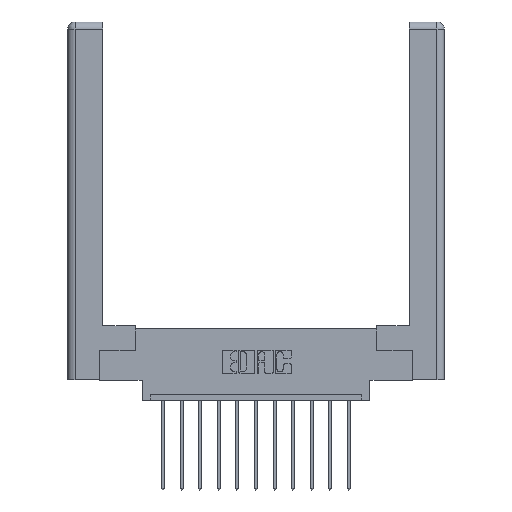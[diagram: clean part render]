
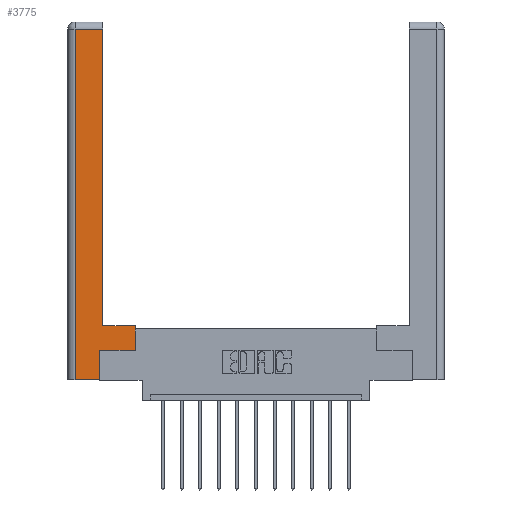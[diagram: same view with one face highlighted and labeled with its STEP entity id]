
A CAD part, top view. The second image highlights one B-rep face of the part: STEP entity #3775.
In plain terms, the highlighted planar face has unit normal (0, 0, 1).
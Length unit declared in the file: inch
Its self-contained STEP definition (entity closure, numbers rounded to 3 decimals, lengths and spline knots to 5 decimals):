
#178 = CARTESIAN_POINT ( 'NONE',  ( 0.295, 2.94, 0. ) ) ;
#1182 = EDGE_CURVE ( 'NONE', #5947, #13692, #11246, .T. ) ;
#1203 = CARTESIAN_POINT ( 'NONE',  ( 0.565, 0.45, 0. ) ) ;
#1439 = CARTESIAN_POINT ( 'NONE',  ( 0.265, 0., 0. ) ) ;
#1519 = FACE_OUTER_BOUND ( 'NONE', #7965, .T. ) ;
#1564 = LINE ( 'NONE', #8539, #3560 ) ;
#1913 = EDGE_CURVE ( 'NONE', #3575, #5947, #8851, .T. ) ;
#1918 = CARTESIAN_POINT ( 'NONE',  ( 0.265, 0.245, 0. ) ) ;
#1952 = VECTOR ( 'NONE', #10999, 39.37008 ) ;
#2088 = VECTOR ( 'NONE', #14551, 39.37008 ) ;
#2549 = VERTEX_POINT ( 'NONE', #10469 ) ;
#3560 = VECTOR ( 'NONE', #7315, 39.37008 ) ;
#3575 = VERTEX_POINT ( 'NONE', #5345 ) ;
#3697 = ORIENTED_EDGE ( 'NONE', *, *, #1182, .T. ) ;
#3775 = ADVANCED_FACE ( 'NONE', ( #1519 ), #8962, .F. ) ;
#3883 = CARTESIAN_POINT ( 'NONE',  ( 0.0615, 0., 0. ) ) ;
#4097 = ORIENTED_EDGE ( 'NONE', *, *, #12690, .T. ) ;
#4231 = VECTOR ( 'NONE', #7386, 39.37008 ) ;
#4236 = DIRECTION ( 'NONE',  ( 0., 1., 0. ) ) ;
#4328 = CARTESIAN_POINT ( 'NONE',  ( 0., 0., 0. ) ) ;
#4984 = LINE ( 'NONE', #7531, #2088 ) ;
#5345 = CARTESIAN_POINT ( 'NONE',  ( 0.265, 0.245, 0. ) ) ;
#5398 = CARTESIAN_POINT ( 'NONE',  ( 0.565, 0.45, 0. ) ) ;
#5839 = EDGE_CURVE ( 'NONE', #7950, #2549, #13059, .T. ) ;
#5947 = VERTEX_POINT ( 'NONE', #10011 ) ;
#6539 = CARTESIAN_POINT ( 'NONE',  ( 0.295, 3., 0. ) ) ;
#6747 = ORIENTED_EDGE ( 'NONE', *, *, #12224, .T. ) ;
#6784 = LINE ( 'NONE', #3883, #4231 ) ;
#7085 = LINE ( 'NONE', #1918, #9625 ) ;
#7102 = VECTOR ( 'NONE', #10967, 39.37008 ) ;
#7315 = DIRECTION ( 'NONE',  ( -1., 0., 0. ) ) ;
#7386 = DIRECTION ( 'NONE',  ( 0., -1., 0. ) ) ;
#7531 = CARTESIAN_POINT ( 'NONE',  ( 0.0615, 2.94, 0. ) ) ;
#7950 = VERTEX_POINT ( 'NONE', #9546 ) ;
#7965 = EDGE_LOOP ( 'NONE', ( #8204, #10056, #6747, #10633, #9139, #12841, #3697, #4097 ) ) ;
#8175 = VECTOR ( 'NONE', #11672, 39.37008 ) ;
#8190 = EDGE_CURVE ( 'NONE', #12531, #10907, #8732, .T. ) ;
#8204 = ORIENTED_EDGE ( 'NONE', *, *, #8190, .T. ) ;
#8539 = CARTESIAN_POINT ( 'NONE',  ( 0.295, 0.45, 0. ) ) ;
#8711 = EDGE_CURVE ( 'NONE', #2549, #3575, #7085, .T. ) ;
#8732 = LINE ( 'NONE', #6539, #7102 ) ;
#8851 = LINE ( 'NONE', #8869, #1952 ) ;
#8869 = CARTESIAN_POINT ( 'NONE',  ( 0.565, 0.245, 0. ) ) ;
#8962 = PLANE ( 'NONE',  #9292 ) ;
#9139 = ORIENTED_EDGE ( 'NONE', *, *, #8711, .T. ) ;
#9292 = AXIS2_PLACEMENT_3D ( 'NONE', #4328, #12459, #13593 ) ;
#9546 = CARTESIAN_POINT ( 'NONE',  ( 0.0615, 0., 0. ) ) ;
#9625 = VECTOR ( 'NONE', #4236, 39.37008 ) ;
#10011 = CARTESIAN_POINT ( 'NONE',  ( 0.565, 0.245, 0. ) ) ;
#10056 = ORIENTED_EDGE ( 'NONE', *, *, #11231, .T. ) ;
#10469 = CARTESIAN_POINT ( 'NONE',  ( 0.265, 0., 0. ) ) ;
#10633 = ORIENTED_EDGE ( 'NONE', *, *, #5839, .T. ) ;
#10780 = DIRECTION ( 'NONE',  ( 1., 0., 0. ) ) ;
#10907 = VERTEX_POINT ( 'NONE', #178 ) ;
#10967 = DIRECTION ( 'NONE',  ( 0., 1., 0. ) ) ;
#10999 = DIRECTION ( 'NONE',  ( 1., 0., 0. ) ) ;
#11112 = VECTOR ( 'NONE', #10780, 39.37008 ) ;
#11231 = EDGE_CURVE ( 'NONE', #10907, #13538, #4984, .T. ) ;
#11246 = LINE ( 'NONE', #1203, #8175 ) ;
#11443 = CARTESIAN_POINT ( 'NONE',  ( 0.295, 0.45, 0. ) ) ;
#11672 = DIRECTION ( 'NONE',  ( 0., 1., 0. ) ) ;
#12224 = EDGE_CURVE ( 'NONE', #13538, #7950, #6784, .T. ) ;
#12459 = DIRECTION ( 'NONE',  ( 0., 0., -1. ) ) ;
#12531 = VERTEX_POINT ( 'NONE', #11443 ) ;
#12690 = EDGE_CURVE ( 'NONE', #13692, #12531, #1564, .T. ) ;
#12841 = ORIENTED_EDGE ( 'NONE', *, *, #1913, .T. ) ;
#13059 = LINE ( 'NONE', #1439, #11112 ) ;
#13245 = CARTESIAN_POINT ( 'NONE',  ( 0.0615, 2.94, 0. ) ) ;
#13538 = VERTEX_POINT ( 'NONE', #13245 ) ;
#13593 = DIRECTION ( 'NONE',  ( -1., 0., 0. ) ) ;
#13692 = VERTEX_POINT ( 'NONE', #5398 ) ;
#14551 = DIRECTION ( 'NONE',  ( -1., 0., 0. ) ) ;
